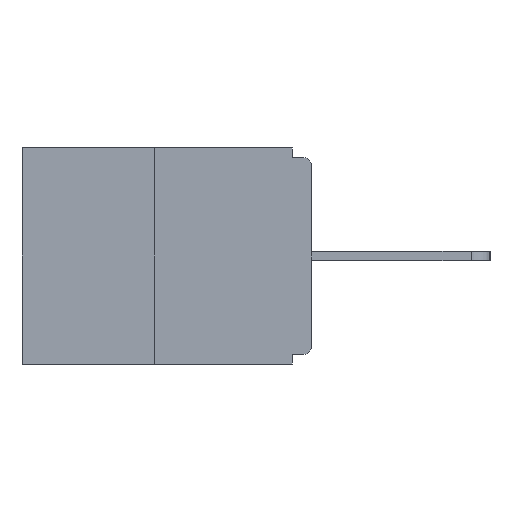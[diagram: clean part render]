
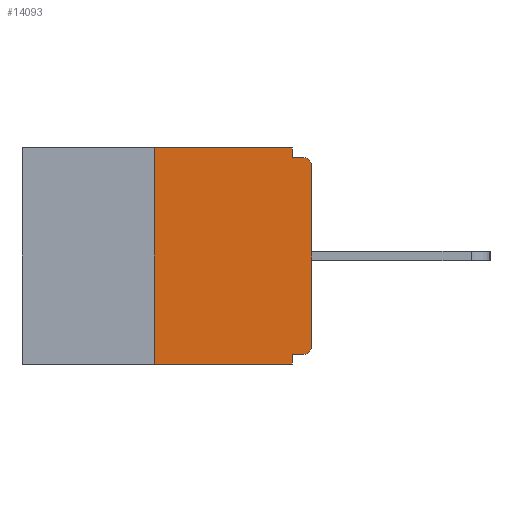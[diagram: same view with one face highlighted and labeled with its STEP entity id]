
A CAD part, left-side view. The second image highlights one B-rep face of the part: STEP entity #14093.
In plain terms, the highlighted planar face has unit normal (-1, 0, 0).
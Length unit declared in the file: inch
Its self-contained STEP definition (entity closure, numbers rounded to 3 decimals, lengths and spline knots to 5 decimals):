
#441 = CARTESIAN_POINT ( 'NONE',  ( 0., 0., -0.015 ) ) ;
#448 = LINE ( 'NONE', #2925, #2389 ) ;
#483 = ORIENTED_EDGE ( 'NONE', *, *, #15803, .F. ) ;
#939 = VERTEX_POINT ( 'NONE', #3334 ) ;
#1121 = PLANE ( 'NONE',  #9122 ) ;
#1590 = DIRECTION ( 'NONE',  ( 0., 0., 1. ) ) ;
#1952 = EDGE_CURVE ( 'NONE', #5254, #8785, #6950, .T. ) ;
#2212 = CARTESIAN_POINT ( 'NONE',  ( 0., 0.031, 0. ) ) ;
#2389 = VECTOR ( 'NONE', #8499, 39.37008 ) ;
#2608 = CARTESIAN_POINT ( 'NONE',  ( 0., 0.031, -0.343 ) ) ;
#2925 = CARTESIAN_POINT ( 'NONE',  ( 0., 0.46, -0.343 ) ) ;
#3334 = CARTESIAN_POINT ( 'NONE',  ( 0., 0.031, -0.328 ) ) ;
#3496 = VECTOR ( 'NONE', #3619, 39.37008 ) ;
#3520 = VECTOR ( 'NONE', #1590, 39.37008 ) ;
#3619 = DIRECTION ( 'NONE',  ( 0., 0., -1. ) ) ;
#3898 = ORIENTED_EDGE ( 'NONE', *, *, #11805, .T. ) ;
#4913 = LINE ( 'NONE', #2212, #3496 ) ;
#5103 = DIRECTION ( 'NONE',  ( 0., 0., -1. ) ) ;
#5171 = DIRECTION ( 'NONE',  ( -1., 0., 0. ) ) ;
#5189 = AXIS2_PLACEMENT_3D ( 'NONE', #9351, #5171, #15726 ) ;
#5254 = VERTEX_POINT ( 'NONE', #8923 ) ;
#5301 = DIRECTION ( 'NONE',  ( 0., 0., -1. ) ) ;
#5317 = CARTESIAN_POINT ( 'NONE',  ( 0., 0.031, -0.015 ) ) ;
#5627 = ORIENTED_EDGE ( 'NONE', *, *, #1952, .T. ) ;
#5957 = CARTESIAN_POINT ( 'NONE',  ( 0., 0.25, -0.343 ) ) ;
#6276 = DIRECTION ( 'NONE',  ( 0., 1., 0. ) ) ;
#6584 = VERTEX_POINT ( 'NONE', #13712 ) ;
#6624 = VERTEX_POINT ( 'NONE', #5957 ) ;
#6950 = LINE ( 'NONE', #16194, #3520 ) ;
#7082 = LINE ( 'NONE', #9509, #14984 ) ;
#7577 = CARTESIAN_POINT ( 'NONE',  ( 0., 0.015, -0.313 ) ) ;
#8043 = DIRECTION ( 'NONE',  ( 0., 0., -1. ) ) ;
#8105 = CARTESIAN_POINT ( 'NONE',  ( 0., 0.031, -0.343 ) ) ;
#8133 = DIRECTION ( 'NONE',  ( 1., 0., 0. ) ) ;
#8384 = DIRECTION ( 'NONE',  ( 0., -1., 0. ) ) ;
#8499 = DIRECTION ( 'NONE',  ( 0., -1., 0. ) ) ;
#8593 = DIRECTION ( 'NONE',  ( 0., 0., 1. ) ) ;
#8747 = ORIENTED_EDGE ( 'NONE', *, *, #11561, .F. ) ;
#8785 = VERTEX_POINT ( 'NONE', #10822 ) ;
#8787 = CIRCLE ( 'NONE', #13248, 0.015 ) ;
#8817 = VERTEX_POINT ( 'NONE', #5317 ) ;
#8825 = CARTESIAN_POINT ( 'NONE',  ( 0., 0.031, 0. ) ) ;
#8923 = CARTESIAN_POINT ( 'NONE',  ( 0., 0., -0.313 ) ) ;
#9046 = CARTESIAN_POINT ( 'NONE',  ( 0., 0., -0.328 ) ) ;
#9122 = AXIS2_PLACEMENT_3D ( 'NONE', #10470, #8133, #8043 ) ;
#9276 = ORIENTED_EDGE ( 'NONE', *, *, #12137, .T. ) ;
#9294 = LINE ( 'NONE', #10610, #13507 ) ;
#9351 = CARTESIAN_POINT ( 'NONE',  ( 0., 0.015, -0.03 ) ) ;
#9509 = CARTESIAN_POINT ( 'NONE',  ( 0., 0.46, 0. ) ) ;
#9720 = EDGE_CURVE ( 'NONE', #6624, #14843, #9294, .T. ) ;
#9881 = VECTOR ( 'NONE', #5301, 39.37008 ) ;
#9952 = EDGE_CURVE ( 'NONE', #13936, #8817, #4913, .T. ) ;
#10392 = VERTEX_POINT ( 'NONE', #2608 ) ;
#10470 = CARTESIAN_POINT ( 'NONE',  ( 0., 0.46, 0. ) ) ;
#10585 = CARTESIAN_POINT ( 'NONE',  ( 0., 0.25, 0. ) ) ;
#10610 = CARTESIAN_POINT ( 'NONE',  ( 0., 0.25, 0. ) ) ;
#10822 = CARTESIAN_POINT ( 'NONE',  ( 0., 0., -0.03 ) ) ;
#11421 = EDGE_CURVE ( 'NONE', #11842, #939, #16996, .T. ) ;
#11561 = EDGE_CURVE ( 'NONE', #939, #10392, #16210, .T. ) ;
#11805 = EDGE_CURVE ( 'NONE', #11842, #5254, #8787, .T. ) ;
#11842 = VERTEX_POINT ( 'NONE', #17062 ) ;
#12137 = EDGE_CURVE ( 'NONE', #6624, #10392, #448, .T. ) ;
#12256 = ORIENTED_EDGE ( 'NONE', *, *, #9952, .F. ) ;
#12331 = EDGE_CURVE ( 'NONE', #8785, #6584, #16883, .T. ) ;
#12783 = EDGE_LOOP ( 'NONE', ( #13684, #13002, #9276, #8747, #13424, #3898, #5627, #15857, #483, #12256 ) ) ;
#12883 = DIRECTION ( 'NONE',  ( -1., 0., 0. ) ) ;
#13002 = ORIENTED_EDGE ( 'NONE', *, *, #9720, .F. ) ;
#13248 = AXIS2_PLACEMENT_3D ( 'NONE', #7577, #12883, #5103 ) ;
#13355 = FACE_OUTER_BOUND ( 'NONE', #12783, .T. ) ;
#13424 = ORIENTED_EDGE ( 'NONE', *, *, #11421, .F. ) ;
#13507 = VECTOR ( 'NONE', #8593, 39.37008 ) ;
#13684 = ORIENTED_EDGE ( 'NONE', *, *, #14193, .F. ) ;
#13712 = CARTESIAN_POINT ( 'NONE',  ( 0., 0.015, -0.015 ) ) ;
#13936 = VERTEX_POINT ( 'NONE', #8825 ) ;
#14073 = LINE ( 'NONE', #441, #16439 ) ;
#14093 = ADVANCED_FACE ( 'NONE', ( #13355 ), #1121, .F. ) ;
#14193 = EDGE_CURVE ( 'NONE', #14843, #13936, #7082, .T. ) ;
#14640 = VECTOR ( 'NONE', #6276, 39.37008 ) ;
#14843 = VERTEX_POINT ( 'NONE', #10585 ) ;
#14984 = VECTOR ( 'NONE', #8384, 39.37008 ) ;
#15293 = DIRECTION ( 'NONE',  ( 0., -1., 0. ) ) ;
#15726 = DIRECTION ( 'NONE',  ( 0., 0., -1. ) ) ;
#15803 = EDGE_CURVE ( 'NONE', #8817, #6584, #14073, .T. ) ;
#15857 = ORIENTED_EDGE ( 'NONE', *, *, #12331, .T. ) ;
#16194 = CARTESIAN_POINT ( 'NONE',  ( 0., 0., 0. ) ) ;
#16210 = LINE ( 'NONE', #8105, #9881 ) ;
#16439 = VECTOR ( 'NONE', #15293, 39.37008 ) ;
#16883 = CIRCLE ( 'NONE', #5189, 0.015 ) ;
#16996 = LINE ( 'NONE', #9046, #14640 ) ;
#17062 = CARTESIAN_POINT ( 'NONE',  ( 0., 0.015, -0.328 ) ) ;
